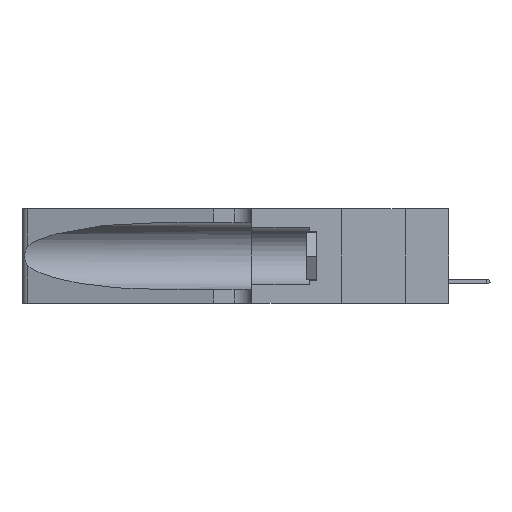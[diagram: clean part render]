
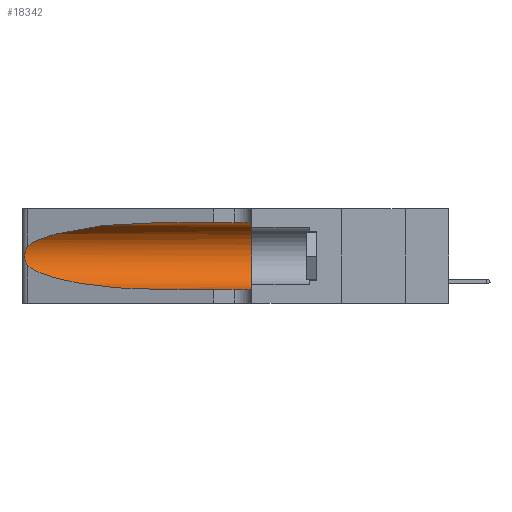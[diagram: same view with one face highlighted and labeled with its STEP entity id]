
A CAD part, left-side view. The second image highlights one B-rep face of the part: STEP entity #18342.
In plain terms, the highlighted cylindrical face has radius 3.308 mm (diameter 6.617 mm), a partial arc.
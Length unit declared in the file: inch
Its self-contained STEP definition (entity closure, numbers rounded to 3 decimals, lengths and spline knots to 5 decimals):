
#878 = CARTESIAN_POINT ( 'NONE',  ( 0.26018, 1.23835, 0.19895 ) ) ;
#1122 = VECTOR ( 'NONE', #22919, 39.37008 ) ;
#1409 = CIRCLE ( 'NONE', #17547, 0.13025 ) ;
#2563 = CARTESIAN_POINT ( 'NONE',  ( 0.18966, 0.96281, 0.05475 ) ) ;
#2628 = ORIENTED_EDGE ( 'NONE', *, *, #21066, .T. ) ;
#3287 = CARTESIAN_POINT ( 'NONE',  ( 0.26075, 1.23896, 0.19203 ) ) ;
#3518 = CARTESIAN_POINT ( 'NONE',  ( 0.25639, 1.23186, 0.15144 ) ) ;
#4458 =( BOUNDED_CURVE ( )  B_SPLINE_CURVE ( 3, ( #31324, #14671, #2563, #29164 ),
 .UNSPECIFIED., .F., .F. ) 
 B_SPLINE_CURVE_WITH_KNOTS ( ( 4, 4 ),
 ( 3.44316, 4.71239 ),
 .UNSPECIFIED. ) 
 CURVE ( )  GEOMETRIC_REPRESENTATION_ITEM ( )  RATIONAL_B_SPLINE_CURVE ( ( 1., 0.87, 0.87, 1. ) ) 
 REPRESENTATION_ITEM ( '' )  );
#5306 = DIRECTION ( 'NONE',  ( 0., 0., 1. ) ) ;
#5561 = CARTESIAN_POINT ( 'NONE',  ( 0.1305, 0.35, 0.31525 ) ) ;
#5595 = CARTESIAN_POINT ( 'NONE',  ( 0.25487, 1.22718, 0.14631 ) ) ;
#5697 = CARTESIAN_POINT ( 'NONE',  ( 0.25856, 1.23593, 0.16098 ) ) ;
#6081 = VERTEX_POINT ( 'NONE', #17355 ) ;
#7200 = DIRECTION ( 'NONE',  ( 0., -1., 0. ) ) ;
#8232 = EDGE_CURVE ( 'NONE', #25836, #6081, #11030, .T. ) ;
#8435 = CARTESIAN_POINT ( 'NONE',  ( 0.1305, 0.35, 0.05475 ) ) ;
#8463 = DIRECTION ( 'NONE',  ( 0., -1., 0. ) ) ;
#8542 = VERTEX_POINT ( 'NONE', #16226 ) ;
#8787 = CARTESIAN_POINT ( 'NONE',  ( 0.1305, 0.72297, 0.31525 ) ) ;
#8821 = EDGE_CURVE ( 'NONE', #25836, #24335, #23945, .T. ) ;
#8943 = VERTEX_POINT ( 'NONE', #12112 ) ;
#9944 = ORIENTED_EDGE ( 'NONE', *, *, #22611, .T. ) ;
#10579 = CARTESIAN_POINT ( 'NONE',  ( 0.25789, 1.23486, 0.15765 ) ) ;
#10712 = EDGE_CURVE ( 'NONE', #24335, #18825, #1409, .T. ) ;
#11030 =( BOUNDED_CURVE ( )  B_SPLINE_CURVE ( 3, ( #8787, #31277, #18995, #21541 ),
 .UNSPECIFIED., .F., .F. ) 
 B_SPLINE_CURVE_WITH_KNOTS ( ( 4, 4 ),
 ( 1.5708, 2.84003 ),
 .UNSPECIFIED. ) 
 CURVE ( )  GEOMETRIC_REPRESENTATION_ITEM ( )  RATIONAL_B_SPLINE_CURVE ( ( 1., 0.87, 0.87, 1. ) ) 
 REPRESENTATION_ITEM ( '' )  );
#12112 = CARTESIAN_POINT ( 'NONE',  ( 0.1305, 0.72297, 0.05475 ) ) ;
#14410 = ORIENTED_EDGE ( 'NONE', *, *, #8232, .T. ) ;
#14671 = CARTESIAN_POINT ( 'NONE',  ( 0.2373, 1.15595, 0.08982 ) ) ;
#15390 = CARTESIAN_POINT ( 'NONE',  ( 0.25555, 1.22994, 0.2215 ) ) ;
#16226 = CARTESIAN_POINT ( 'NONE',  ( 0.25487, 1.22718, 0.14631 ) ) ;
#17355 = CARTESIAN_POINT ( 'NONE',  ( 0.25487, 1.22718, 0.22369 ) ) ;
#17434 = DIRECTION ( 'NONE',  ( 0., 1., 0. ) ) ;
#17547 = AXIS2_PLACEMENT_3D ( 'NONE', #29592, #17434, #5306 ) ;
#17718 = CARTESIAN_POINT ( 'NONE',  ( 0.25555, 1.22993, 0.14849 ) ) ;
#17826 = CARTESIAN_POINT ( 'NONE',  ( 0.25787, 1.23484, 0.2124 ) ) ;
#18048 = CARTESIAN_POINT ( 'NONE',  ( 0.25854, 1.2359, 0.20912 ) ) ;
#18342 = ADVANCED_FACE ( 'NONE', ( #31325 ), #18717, .F. ) ;
#18717 = CYLINDRICAL_SURFACE ( 'NONE', #20953, 0.13025 ) ;
#18825 = VERTEX_POINT ( 'NONE', #8435 ) ;
#18995 = CARTESIAN_POINT ( 'NONE',  ( 0.2373, 1.15595, 0.28018 ) ) ;
#19298 = CARTESIAN_POINT ( 'NONE',  ( 0.1305, 0.72297, 0.31525 ) ) ;
#20160 = CARTESIAN_POINT ( 'NONE',  ( 0.25487, 1.22718, 0.22369 ) ) ;
#20271 = ORIENTED_EDGE ( 'NONE', *, *, #10712, .F. ) ;
#20276 = CARTESIAN_POINT ( 'NONE',  ( 0.26017, 1.23833, 0.17102 ) ) ;
#20341 = CARTESIAN_POINT ( 'NONE',  ( 0.1305, 1.61858, 0.31525 ) ) ;
#20545 = VECTOR ( 'NONE', #7200, 39.37008 ) ;
#20741 = ORIENTED_EDGE ( 'NONE', *, *, #27539, .T. ) ;
#20953 = AXIS2_PLACEMENT_3D ( 'NONE', #23081, #8463, #27985 ) ;
#20964 = B_SPLINE_CURVE_WITH_KNOTS ( 'NONE', 3,
 ( #20160, #15390, #22743, #17826, #18048, #878, #3287, #25232, #20276, #5697, #10579, #3518, #17718, #5595 ),
 .UNSPECIFIED., .F., .F.,
 ( 4, 2, 2, 2, 2, 2, 4 ),
 ( 0., 0.00027, 0.00053, 0.00107, 0.0016, 0.00187, 0.00214 ),
 .UNSPECIFIED. ) ;
#21066 = EDGE_CURVE ( 'NONE', #8542, #8943, #4458, .T. ) ;
#21187 = EDGE_LOOP ( 'NONE', ( #14410, #20741, #2628, #9944, #20271, #30128 ) ) ;
#21541 = CARTESIAN_POINT ( 'NONE',  ( 0.25487, 1.22718, 0.22369 ) ) ;
#22611 = EDGE_CURVE ( 'NONE', #8943, #18825, #29337, .T. ) ;
#22743 = CARTESIAN_POINT ( 'NONE',  ( 0.25639, 1.23184, 0.21858 ) ) ;
#22919 = DIRECTION ( 'NONE',  ( 0., -1., 0. ) ) ;
#23081 = CARTESIAN_POINT ( 'NONE',  ( 0.1305, 1.61858, 0.185 ) ) ;
#23532 = CARTESIAN_POINT ( 'NONE',  ( 0.1305, 1.61858, 0.05475 ) ) ;
#23945 = LINE ( 'NONE', #20341, #1122 ) ;
#24335 = VERTEX_POINT ( 'NONE', #5561 ) ;
#25232 = CARTESIAN_POINT ( 'NONE',  ( 0.26075, 1.23896, 0.178 ) ) ;
#25836 = VERTEX_POINT ( 'NONE', #19298 ) ;
#27539 = EDGE_CURVE ( 'NONE', #6081, #8542, #20964, .T. ) ;
#27985 = DIRECTION ( 'NONE',  ( 0., 0., -1. ) ) ;
#29164 = CARTESIAN_POINT ( 'NONE',  ( 0.1305, 0.72297, 0.05475 ) ) ;
#29337 = LINE ( 'NONE', #23532, #20545 ) ;
#29592 = CARTESIAN_POINT ( 'NONE',  ( 0.1305, 0.35, 0.185 ) ) ;
#30128 = ORIENTED_EDGE ( 'NONE', *, *, #8821, .F. ) ;
#31277 = CARTESIAN_POINT ( 'NONE',  ( 0.18966, 0.96281, 0.31525 ) ) ;
#31324 = CARTESIAN_POINT ( 'NONE',  ( 0.25487, 1.22718, 0.14631 ) ) ;
#31325 = FACE_OUTER_BOUND ( 'NONE', #21187, .T. ) ;
